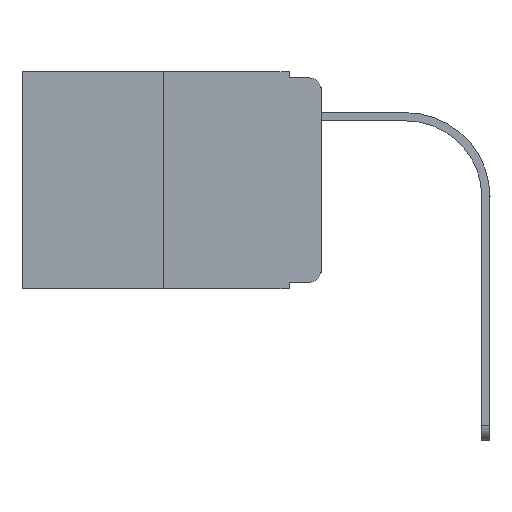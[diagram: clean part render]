
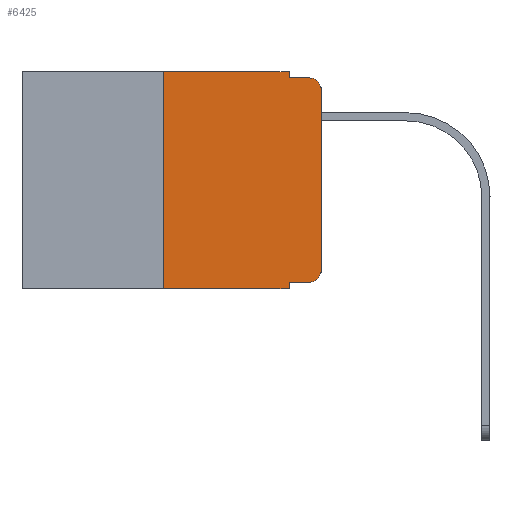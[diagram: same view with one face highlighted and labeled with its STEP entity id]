
A CAD part, left-side view. The second image highlights one B-rep face of the part: STEP entity #6425.
In plain terms, the highlighted planar face has unit normal (-1, 0, 0).
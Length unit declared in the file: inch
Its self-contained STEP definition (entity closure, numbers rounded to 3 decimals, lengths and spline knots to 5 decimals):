
#87 = DIRECTION ( 'NONE',  ( 0., -1., 0. ) ) ;
#540 = CARTESIAN_POINT ( 'NONE',  ( 0., 0.051, 0. ) ) ;
#889 = VERTEX_POINT ( 'NONE', #7102 ) ;
#2014 = CARTESIAN_POINT ( 'NONE',  ( 0., 0.02, -0.313 ) ) ;
#2065 = CARTESIAN_POINT ( 'NONE',  ( 0., 0.473, -0.343 ) ) ;
#2100 = CARTESIAN_POINT ( 'NONE',  ( 0., 0.051, -0.333 ) ) ;
#2142 = VERTEX_POINT ( 'NONE', #21467 ) ;
#3171 = DIRECTION ( 'NONE',  ( 0., 0., -1. ) ) ;
#3178 = CARTESIAN_POINT ( 'NONE',  ( 0., 0.051, -0.01 ) ) ;
#3872 = VECTOR ( 'NONE', #19486, 39.37008 ) ;
#4089 = VERTEX_POINT ( 'NONE', #9946 ) ;
#4239 = DIRECTION ( 'NONE',  ( 0., -1., 0. ) ) ;
#4389 = EDGE_CURVE ( 'NONE', #22396, #11446, #8786, .T. ) ;
#4403 = VECTOR ( 'NONE', #22356, 39.37008 ) ;
#4586 = CARTESIAN_POINT ( 'NONE',  ( 0., 0.25, -0.343 ) ) ;
#4802 = LINE ( 'NONE', #540, #4403 ) ;
#4915 = EDGE_LOOP ( 'NONE', ( #5825, #20312, #8669, #8279, #13950, #20244, #17134, #11174, #20856, #8473 ) ) ;
#4941 = CARTESIAN_POINT ( 'NONE',  ( 0., 0.02, -0.01 ) ) ;
#5825 = ORIENTED_EDGE ( 'NONE', *, *, #6613, .T. ) ;
#6246 = CARTESIAN_POINT ( 'NONE',  ( 0., 0., -0.313 ) ) ;
#6319 = VECTOR ( 'NONE', #7991, 39.37008 ) ;
#6425 = ADVANCED_FACE ( 'NONE', ( #11585 ), #9269, .F. ) ;
#6613 = EDGE_CURVE ( 'NONE', #11274, #22396, #12348, .T. ) ;
#7102 = CARTESIAN_POINT ( 'NONE',  ( 0., 0.051, 0. ) ) ;
#7460 = CARTESIAN_POINT ( 'NONE',  ( 0., 0.02, -0.03 ) ) ;
#7799 = EDGE_CURVE ( 'NONE', #12298, #11446, #8372, .T. ) ;
#7815 = VERTEX_POINT ( 'NONE', #24262 ) ;
#7991 = DIRECTION ( 'NONE',  ( 0., 0., 1. ) ) ;
#8279 = ORIENTED_EDGE ( 'NONE', *, *, #23886, .F. ) ;
#8372 = LINE ( 'NONE', #20008, #20384 ) ;
#8473 = ORIENTED_EDGE ( 'NONE', *, *, #25374, .T. ) ;
#8669 = ORIENTED_EDGE ( 'NONE', *, *, #7799, .F. ) ;
#8691 = EDGE_CURVE ( 'NONE', #10993, #4089, #19237, .T. ) ;
#8786 = CIRCLE ( 'NONE', #18269, 0.02 ) ;
#9242 = VECTOR ( 'NONE', #3171, 39.37008 ) ;
#9269 = PLANE ( 'NONE',  #17604 ) ;
#9367 = EDGE_CURVE ( 'NONE', #20420, #889, #13897, .T. ) ;
#9468 = DIRECTION ( 'NONE',  ( 0., 0., -1. ) ) ;
#9794 = CARTESIAN_POINT ( 'NONE',  ( 0., 0., 0. ) ) ;
#9946 = CARTESIAN_POINT ( 'NONE',  ( 0., 0.051, -0.343 ) ) ;
#10102 = LINE ( 'NONE', #2100, #15698 ) ;
#10993 = VERTEX_POINT ( 'NONE', #4586 ) ;
#11174 = ORIENTED_EDGE ( 'NONE', *, *, #11866, .F. ) ;
#11274 = VERTEX_POINT ( 'NONE', #6246 ) ;
#11446 = VERTEX_POINT ( 'NONE', #4941 ) ;
#11585 = FACE_OUTER_BOUND ( 'NONE', #4915, .T. ) ;
#11799 = CARTESIAN_POINT ( 'NONE',  ( 0., 0., -0.03 ) ) ;
#11866 = EDGE_CURVE ( 'NONE', #7815, #4089, #4802, .T. ) ;
#12298 = VERTEX_POINT ( 'NONE', #3178 ) ;
#12348 = LINE ( 'NONE', #9794, #6319 ) ;
#12421 = CARTESIAN_POINT ( 'NONE',  ( 0., 0.25, 0. ) ) ;
#12932 = EDGE_CURVE ( 'NONE', #7815, #2142, #10102, .T. ) ;
#13868 = DIRECTION ( 'NONE',  ( -1., 0., 0. ) ) ;
#13897 = LINE ( 'NONE', #22286, #15865 ) ;
#13950 = ORIENTED_EDGE ( 'NONE', *, *, #9367, .F. ) ;
#14131 = VECTOR ( 'NONE', #22377, 39.37008 ) ;
#14657 = LINE ( 'NONE', #22919, #9242 ) ;
#15698 = VECTOR ( 'NONE', #23660, 39.37008 ) ;
#15865 = VECTOR ( 'NONE', #87, 39.37008 ) ;
#17134 = ORIENTED_EDGE ( 'NONE', *, *, #8691, .T. ) ;
#17402 = CARTESIAN_POINT ( 'NONE',  ( 0., 0.473, 0. ) ) ;
#17578 = CIRCLE ( 'NONE', #24186, 0.02 ) ;
#17604 = AXIS2_PLACEMENT_3D ( 'NONE', #17402, #19083, #21014 ) ;
#18269 = AXIS2_PLACEMENT_3D ( 'NONE', #7460, #19468, #23359 ) ;
#19083 = DIRECTION ( 'NONE',  ( 1., 0., 0. ) ) ;
#19237 = LINE ( 'NONE', #2065, #3872 ) ;
#19468 = DIRECTION ( 'NONE',  ( -1., 0., 0. ) ) ;
#19486 = DIRECTION ( 'NONE',  ( 0., -1., 0. ) ) ;
#20008 = CARTESIAN_POINT ( 'NONE',  ( 0., 0.051, -0.01 ) ) ;
#20244 = ORIENTED_EDGE ( 'NONE', *, *, #22551, .F. ) ;
#20312 = ORIENTED_EDGE ( 'NONE', *, *, #4389, .T. ) ;
#20384 = VECTOR ( 'NONE', #4239, 39.37008 ) ;
#20420 = VERTEX_POINT ( 'NONE', #20532 ) ;
#20532 = CARTESIAN_POINT ( 'NONE',  ( 0., 0.25, 0. ) ) ;
#20856 = ORIENTED_EDGE ( 'NONE', *, *, #12932, .T. ) ;
#21014 = DIRECTION ( 'NONE',  ( 0., 0., -1. ) ) ;
#21467 = CARTESIAN_POINT ( 'NONE',  ( 0., 0.02, -0.333 ) ) ;
#22286 = CARTESIAN_POINT ( 'NONE',  ( 0., 0.473, 0. ) ) ;
#22356 = DIRECTION ( 'NONE',  ( 0., 0., -1. ) ) ;
#22377 = DIRECTION ( 'NONE',  ( 0., 0., 1. ) ) ;
#22396 = VERTEX_POINT ( 'NONE', #11799 ) ;
#22516 = LINE ( 'NONE', #12421, #14131 ) ;
#22551 = EDGE_CURVE ( 'NONE', #10993, #20420, #22516, .T. ) ;
#22919 = CARTESIAN_POINT ( 'NONE',  ( 0., 0.051, 0. ) ) ;
#23359 = DIRECTION ( 'NONE',  ( 0., 0., -1. ) ) ;
#23660 = DIRECTION ( 'NONE',  ( 0., -1., 0. ) ) ;
#23886 = EDGE_CURVE ( 'NONE', #889, #12298, #14657, .T. ) ;
#24186 = AXIS2_PLACEMENT_3D ( 'NONE', #2014, #13868, #9468 ) ;
#24262 = CARTESIAN_POINT ( 'NONE',  ( 0., 0.051, -0.333 ) ) ;
#25374 = EDGE_CURVE ( 'NONE', #2142, #11274, #17578, .T. ) ;
